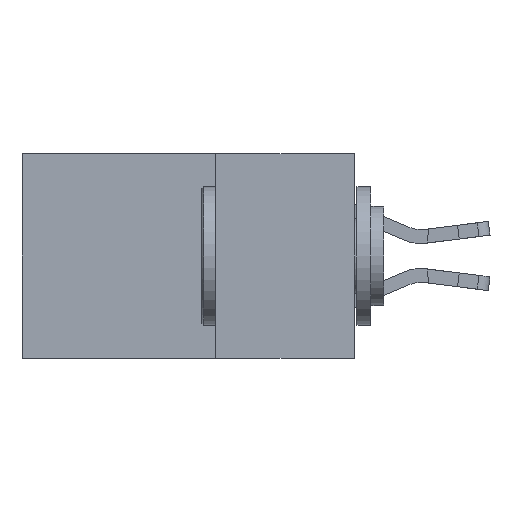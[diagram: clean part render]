
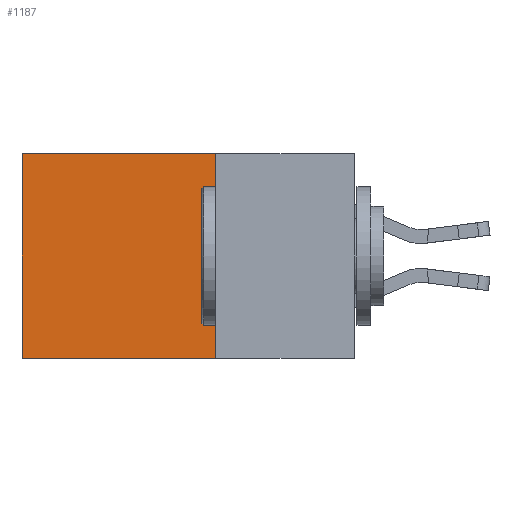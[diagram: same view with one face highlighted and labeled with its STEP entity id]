
A CAD part, left-side view. The second image highlights one B-rep face of the part: STEP entity #1187.
In plain terms, the highlighted planar face has unit normal (-1, 0, 0).
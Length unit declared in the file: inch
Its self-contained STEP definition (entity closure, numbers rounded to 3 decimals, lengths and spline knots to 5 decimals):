
#6 = LINE ( 'NONE', #4467, #6105 ) ;
#68 = EDGE_CURVE ( 'NONE', #7686, #12580, #12117, .T. ) ;
#1187 = ADVANCED_FACE ( 'NONE', ( #5592 ), #4277, .F. ) ;
#1622 = DIRECTION ( 'NONE',  ( 0., 0., -1. ) ) ;
#2500 = AXIS2_PLACEMENT_3D ( 'NONE', #2724, #3138, #1622 ) ;
#2724 = CARTESIAN_POINT ( 'NONE',  ( 0.298, 0.25, 0. ) ) ;
#3138 = DIRECTION ( 'NONE',  ( 1., 0., 0. ) ) ;
#3179 = VERTEX_POINT ( 'NONE', #6084 ) ;
#3658 = CARTESIAN_POINT ( 'NONE',  ( 0.298, 0.25, 0. ) ) ;
#4277 = PLANE ( 'NONE',  #2500 ) ;
#4467 = CARTESIAN_POINT ( 'NONE',  ( 0.298, 0.6, 0. ) ) ;
#4616 = VECTOR ( 'NONE', #11550, 39.37008 ) ;
#5197 = CARTESIAN_POINT ( 'NONE',  ( 0.298, 0.25, -0.37 ) ) ;
#5359 = ORIENTED_EDGE ( 'NONE', *, *, #8901, .T. ) ;
#5592 = FACE_OUTER_BOUND ( 'NONE', #7863, .T. ) ;
#5877 = EDGE_CURVE ( 'NONE', #7332, #3179, #12119, .T. ) ;
#6051 = LINE ( 'NONE', #3658, #4616 ) ;
#6084 = CARTESIAN_POINT ( 'NONE',  ( 0.298, 0.6, -0.37 ) ) ;
#6105 = VECTOR ( 'NONE', #12762, 39.37008 ) ;
#6166 = VECTOR ( 'NONE', #11116, 39.37008 ) ;
#6645 = CARTESIAN_POINT ( 'NONE',  ( 0.298, 0.6, 0. ) ) ;
#7332 = VERTEX_POINT ( 'NONE', #13793 ) ;
#7558 = CARTESIAN_POINT ( 'NONE',  ( 0.298, 0.25, 0. ) ) ;
#7629 = CARTESIAN_POINT ( 'NONE',  ( 0.298, 0.25, 0. ) ) ;
#7686 = VERTEX_POINT ( 'NONE', #7558 ) ;
#7863 = EDGE_LOOP ( 'NONE', ( #5359, #10928, #7930, #12573 ) ) ;
#7930 = ORIENTED_EDGE ( 'NONE', *, *, #10728, .F. ) ;
#8901 = EDGE_CURVE ( 'NONE', #12580, #3179, #6, .T. ) ;
#9798 = DIRECTION ( 'NONE',  ( 0., 1., 0. ) ) ;
#10728 = EDGE_CURVE ( 'NONE', #7686, #7332, #6051, .T. ) ;
#10928 = ORIENTED_EDGE ( 'NONE', *, *, #5877, .F. ) ;
#11116 = DIRECTION ( 'NONE',  ( 0., 1., 0. ) ) ;
#11550 = DIRECTION ( 'NONE',  ( 0., 0., -1. ) ) ;
#12117 = LINE ( 'NONE', #7629, #6166 ) ;
#12119 = LINE ( 'NONE', #5197, #12623 ) ;
#12573 = ORIENTED_EDGE ( 'NONE', *, *, #68, .T. ) ;
#12580 = VERTEX_POINT ( 'NONE', #6645 ) ;
#12623 = VECTOR ( 'NONE', #9798, 39.37008 ) ;
#12762 = DIRECTION ( 'NONE',  ( 0., 0., -1. ) ) ;
#13793 = CARTESIAN_POINT ( 'NONE',  ( 0.298, 0.25, -0.37 ) ) ;
